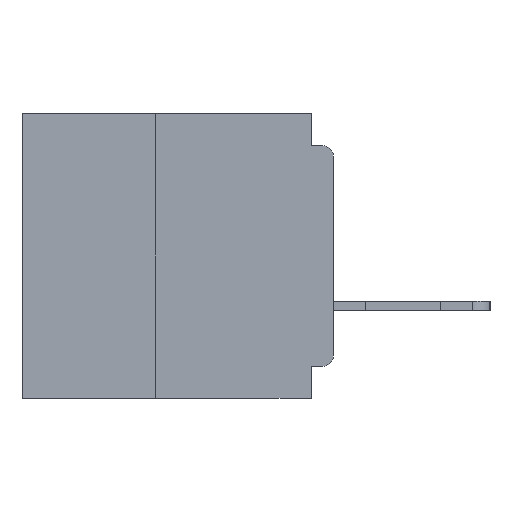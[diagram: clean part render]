
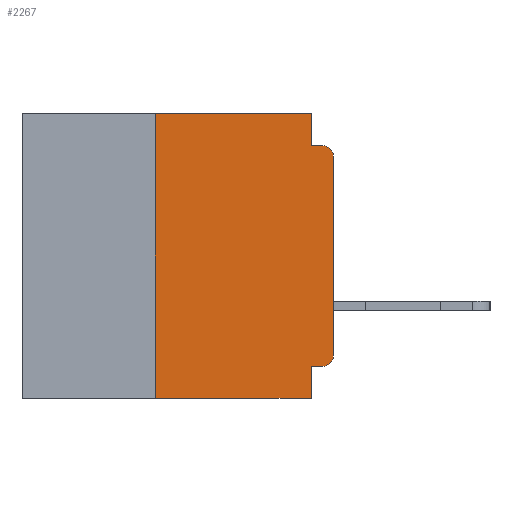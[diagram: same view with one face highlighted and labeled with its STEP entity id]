
A CAD part, left-side view. The second image highlights one B-rep face of the part: STEP entity #2267.
In plain terms, the highlighted planar face has unit normal (-1, 0, 0).
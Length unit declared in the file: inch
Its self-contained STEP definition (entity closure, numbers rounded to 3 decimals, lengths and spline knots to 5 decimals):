
#431 = CARTESIAN_POINT ( 'NONE',  ( 0., 0.015, -0.06 ) ) ;
#1019 = EDGE_CURVE ( 'NONE', #9022, #21159, #24127, .T. ) ;
#1699 = DIRECTION ( 'NONE',  ( 0., 0., 1. ) ) ;
#2267 = ADVANCED_FACE ( 'NONE', ( #15355 ), #25050, .F. ) ;
#2755 = LINE ( 'NONE', #25286, #11422 ) ;
#3680 = CARTESIAN_POINT ( 'NONE',  ( 0., 0.437, -0.4 ) ) ;
#4167 = DIRECTION ( 'NONE',  ( 0., 0., -1. ) ) ;
#5162 = DIRECTION ( 'NONE',  ( 0., 0., -1. ) ) ;
#8142 = ORIENTED_EDGE ( 'NONE', *, *, #46864, .F. ) ;
#8273 = CARTESIAN_POINT ( 'NONE',  ( 0., 0., -0.34 ) ) ;
#8837 = CARTESIAN_POINT ( 'NONE',  ( 0., 0.015, -0.355 ) ) ;
#8902 = EDGE_CURVE ( 'NONE', #19114, #9527, #17665, .T. ) ;
#9022 = VERTEX_POINT ( 'NONE', #8837 ) ;
#9431 = EDGE_CURVE ( 'NONE', #21159, #19072, #32619, .T. ) ;
#9527 = VERTEX_POINT ( 'NONE', #22674 ) ;
#9695 = CARTESIAN_POINT ( 'NONE',  ( 0., 0.25, 0. ) ) ;
#10460 = ORIENTED_EDGE ( 'NONE', *, *, #24662, .F. ) ;
#11307 = DIRECTION ( 'NONE',  ( -1., 0., 0. ) ) ;
#11422 = VECTOR ( 'NONE', #29000, 39.37008 ) ;
#11900 = DIRECTION ( 'NONE',  ( 0., -1., 0. ) ) ;
#12441 = VECTOR ( 'NONE', #1699, 39.37008 ) ;
#12823 = LINE ( 'NONE', #3680, #21476 ) ;
#13078 = DIRECTION ( 'NONE',  ( 0., -1., 0. ) ) ;
#13151 = CARTESIAN_POINT ( 'NONE',  ( 0., 0.031, -0.045 ) ) ;
#13672 = EDGE_CURVE ( 'NONE', #43686, #19072, #12823, .T. ) ;
#14971 = CARTESIAN_POINT ( 'NONE',  ( 0., 0., -0.06 ) ) ;
#15355 = FACE_OUTER_BOUND ( 'NONE', #21260, .T. ) ;
#17270 = CARTESIAN_POINT ( 'NONE',  ( 0., 0.25, -0.4 ) ) ;
#17330 = CARTESIAN_POINT ( 'NONE',  ( 0., 0.031, 0. ) ) ;
#17606 = LINE ( 'NONE', #46236, #44680 ) ;
#17655 = DIRECTION ( 'NONE',  ( 0., 1., 0. ) ) ;
#17665 = LINE ( 'NONE', #37668, #45884 ) ;
#19072 = VERTEX_POINT ( 'NONE', #31543 ) ;
#19114 = VERTEX_POINT ( 'NONE', #13151 ) ;
#19170 = VERTEX_POINT ( 'NONE', #17330 ) ;
#19655 = ORIENTED_EDGE ( 'NONE', *, *, #34797, .T. ) ;
#21159 = VERTEX_POINT ( 'NONE', #25721 ) ;
#21187 = CIRCLE ( 'NONE', #24914, 0.015 ) ;
#21260 = EDGE_LOOP ( 'NONE', ( #33462, #44409, #38070, #34056, #8142, #10460, #30065, #41007, #34643, #19655 ) ) ;
#21476 = VECTOR ( 'NONE', #22064, 39.37008 ) ;
#22064 = DIRECTION ( 'NONE',  ( 0., -1., 0. ) ) ;
#22674 = CARTESIAN_POINT ( 'NONE',  ( 0., 0.015, -0.045 ) ) ;
#23833 = CARTESIAN_POINT ( 'NONE',  ( 0., 0.25, -0.4 ) ) ;
#24127 = LINE ( 'NONE', #26341, #42539 ) ;
#24662 = EDGE_CURVE ( 'NONE', #43686, #37940, #40722, .T. ) ;
#24914 = AXIS2_PLACEMENT_3D ( 'NONE', #33366, #11307, #37071 ) ;
#25050 = PLANE ( 'NONE',  #40626 ) ;
#25286 = CARTESIAN_POINT ( 'NONE',  ( 0., 0.031, 0. ) ) ;
#25597 = EDGE_CURVE ( 'NONE', #40745, #38209, #37149, .T. ) ;
#25721 = CARTESIAN_POINT ( 'NONE',  ( 0., 0.031, -0.355 ) ) ;
#25907 = DIRECTION ( 'NONE',  ( 1., 0., 0. ) ) ;
#26053 = DIRECTION ( 'NONE',  ( 0., 0., -1. ) ) ;
#26268 = DIRECTION ( 'NONE',  ( -1., 0., 0. ) ) ;
#26341 = CARTESIAN_POINT ( 'NONE',  ( 0., 0., -0.355 ) ) ;
#26579 = CARTESIAN_POINT ( 'NONE',  ( 0., 0.437, 0. ) ) ;
#29000 = DIRECTION ( 'NONE',  ( 0., 0., -1. ) ) ;
#29708 = CIRCLE ( 'NONE', #46261, 0.015 ) ;
#30065 = ORIENTED_EDGE ( 'NONE', *, *, #13672, .T. ) ;
#31543 = CARTESIAN_POINT ( 'NONE',  ( 0., 0.031, -0.4 ) ) ;
#32619 = LINE ( 'NONE', #36838, #40103 ) ;
#33366 = CARTESIAN_POINT ( 'NONE',  ( 0., 0.015, -0.34 ) ) ;
#33462 = ORIENTED_EDGE ( 'NONE', *, *, #25597, .T. ) ;
#34056 = ORIENTED_EDGE ( 'NONE', *, *, #45509, .F. ) ;
#34643 = ORIENTED_EDGE ( 'NONE', *, *, #1019, .F. ) ;
#34797 = EDGE_CURVE ( 'NONE', #9022, #40745, #21187, .T. ) ;
#35994 = VECTOR ( 'NONE', #36288, 39.37008 ) ;
#36288 = DIRECTION ( 'NONE',  ( 0., 0., 1. ) ) ;
#36838 = CARTESIAN_POINT ( 'NONE',  ( 0., 0.031, -0.4 ) ) ;
#37071 = DIRECTION ( 'NONE',  ( 0., 0., -1. ) ) ;
#37149 = LINE ( 'NONE', #43693, #35994 ) ;
#37668 = CARTESIAN_POINT ( 'NONE',  ( 0., 0., -0.045 ) ) ;
#37940 = VERTEX_POINT ( 'NONE', #9695 ) ;
#38070 = ORIENTED_EDGE ( 'NONE', *, *, #8902, .F. ) ;
#38209 = VERTEX_POINT ( 'NONE', #14971 ) ;
#40103 = VECTOR ( 'NONE', #26053, 39.37008 ) ;
#40626 = AXIS2_PLACEMENT_3D ( 'NONE', #26579, #25907, #5162 ) ;
#40722 = LINE ( 'NONE', #23833, #12441 ) ;
#40745 = VERTEX_POINT ( 'NONE', #8273 ) ;
#41007 = ORIENTED_EDGE ( 'NONE', *, *, #9431, .F. ) ;
#42539 = VECTOR ( 'NONE', #17655, 39.37008 ) ;
#43686 = VERTEX_POINT ( 'NONE', #17270 ) ;
#43693 = CARTESIAN_POINT ( 'NONE',  ( 0., 0., 0. ) ) ;
#44409 = ORIENTED_EDGE ( 'NONE', *, *, #47199, .T. ) ;
#44680 = VECTOR ( 'NONE', #13078, 39.37008 ) ;
#45509 = EDGE_CURVE ( 'NONE', #19170, #19114, #2755, .T. ) ;
#45884 = VECTOR ( 'NONE', #11900, 39.37008 ) ;
#46236 = CARTESIAN_POINT ( 'NONE',  ( 0., 0.437, 0. ) ) ;
#46261 = AXIS2_PLACEMENT_3D ( 'NONE', #431, #26268, #4167 ) ;
#46864 = EDGE_CURVE ( 'NONE', #37940, #19170, #17606, .T. ) ;
#47199 = EDGE_CURVE ( 'NONE', #38209, #9527, #29708, .T. ) ;
